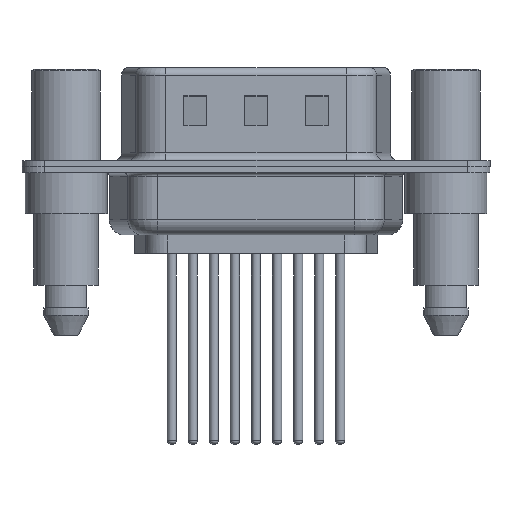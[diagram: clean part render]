
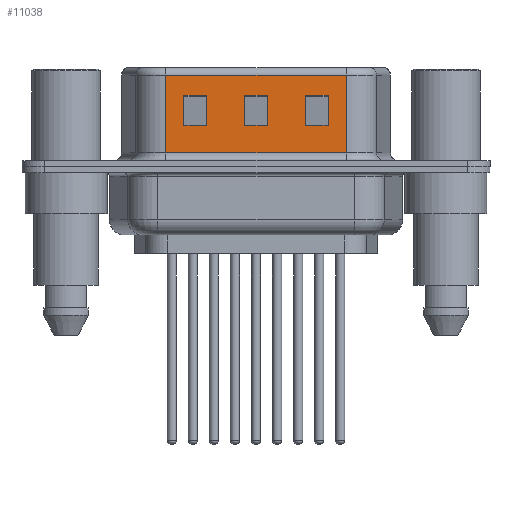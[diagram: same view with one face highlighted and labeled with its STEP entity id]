
A CAD part, front view. The second image highlights one B-rep face of the part: STEP entity #11038.
In plain terms, the highlighted planar face has unit normal (0, -1, 0).
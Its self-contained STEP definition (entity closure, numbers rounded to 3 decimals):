
#74 = CARTESIAN_POINT ( 'NONE',  ( 9.25, -4.55, 4.705 ) ) ;
#167 = CARTESIAN_POINT ( 'NONE',  ( 17.25, -4.55, 6.52 ) ) ;
#436 = LINE ( 'NONE', #4995, #13850 ) ;
#758 = VERTEX_POINT ( 'NONE', #74 ) ;
#816 = ORIENTED_EDGE ( 'NONE', *, *, #9312, .T. ) ;
#884 = VECTOR ( 'NONE', #4699, 1000. ) ;
#929 = VECTOR ( 'NONE', #10079, 1000. ) ;
#950 = DIRECTION ( 'NONE',  ( 0., 0., -1. ) ) ;
#968 = DIRECTION ( 'NONE',  ( -1., 0., 0. ) ) ;
#1068 = EDGE_CURVE ( 'NONE', #1913, #12412, #10161, .T. ) ;
#1203 = DIRECTION ( 'NONE',  ( 0., 0., -1. ) ) ;
#1407 = CARTESIAN_POINT ( 'NONE',  ( 18.451, -4.55, 0.9 ) ) ;
#1433 = VERTEX_POINT ( 'NONE', #2046 ) ;
#1436 = VECTOR ( 'NONE', #12580, 1000. ) ;
#1450 = VERTEX_POINT ( 'NONE', #7781 ) ;
#1588 = EDGE_LOOP ( 'NONE', ( #8142, #12219, #5133, #12017 ) ) ;
#1843 = EDGE_CURVE ( 'NONE', #12696, #6609, #7692, .T. ) ;
#1893 = ORIENTED_EDGE ( 'NONE', *, *, #9123, .T. ) ;
#1907 = EDGE_CURVE ( 'NONE', #1450, #7329, #2392, .T. ) ;
#1913 = VERTEX_POINT ( 'NONE', #11453 ) ;
#1971 = VECTOR ( 'NONE', #6741, 1000. ) ;
#2046 = CARTESIAN_POINT ( 'NONE',  ( 17.25, -4.55, 4.705 ) ) ;
#2392 = LINE ( 'NONE', #5786, #5528 ) ;
#2848 = VECTOR ( 'NONE', #13832, 1000. ) ;
#2907 = ORIENTED_EDGE ( 'NONE', *, *, #3967, .T. ) ;
#3003 = EDGE_CURVE ( 'NONE', #5905, #1450, #13193, .T. ) ;
#3876 = VECTOR ( 'NONE', #14158, 1000. ) ;
#3967 = EDGE_CURVE ( 'NONE', #9337, #12696, #13214, .T. ) ;
#4340 = CARTESIAN_POINT ( 'NONE',  ( 15.75, -4.55, 6.52 ) ) ;
#4435 = VERTEX_POINT ( 'NONE', #8905 ) ;
#4531 = AXIS2_PLACEMENT_3D ( 'NONE', #6543, #13302, #6613 ) ;
#4615 = EDGE_CURVE ( 'NONE', #1913, #10646, #9132, .T. ) ;
#4657 = VERTEX_POINT ( 'NONE', #8022 ) ;
#4660 = DIRECTION ( 'NONE',  ( 1., 0., 0. ) ) ;
#4699 = DIRECTION ( 'NONE',  ( -1., 0., 0. ) ) ;
#4855 = LINE ( 'NONE', #9362, #2848 ) ;
#4920 = DIRECTION ( 'NONE',  ( 1., 0., 0. ) ) ;
#4995 = CARTESIAN_POINT ( 'NONE',  ( 14.451, -4.55, 4.705 ) ) ;
#5128 = CARTESIAN_POINT ( 'NONE',  ( 7.75, -4.55, 4.705 ) ) ;
#5133 = ORIENTED_EDGE ( 'NONE', *, *, #3003, .T. ) ;
#5211 = CARTESIAN_POINT ( 'NONE',  ( 6.549, -4.55, 0.9 ) ) ;
#5231 = LINE ( 'NONE', #9727, #14067 ) ;
#5528 = VECTOR ( 'NONE', #6887, 1000. ) ;
#5719 = EDGE_CURVE ( 'NONE', #11653, #4657, #5231, .T. ) ;
#5736 = ORIENTED_EDGE ( 'NONE', *, *, #6155, .T. ) ;
#5747 = CARTESIAN_POINT ( 'NONE',  ( 18.451, -4.55, 6.02 ) ) ;
#5786 = CARTESIAN_POINT ( 'NONE',  ( 11.75, -4.55, 6.52 ) ) ;
#5815 = VECTOR ( 'NONE', #9989, 1000. ) ;
#5905 = VERTEX_POINT ( 'NONE', #6856 ) ;
#5963 = VECTOR ( 'NONE', #4660, 1000. ) ;
#6142 = VERTEX_POINT ( 'NONE', #9570 ) ;
#6155 = EDGE_CURVE ( 'NONE', #6609, #758, #436, .T. ) ;
#6403 = EDGE_CURVE ( 'NONE', #758, #9337, #13445, .T. ) ;
#6543 = CARTESIAN_POINT ( 'NONE',  ( 18.451, -4.55, 6.52 ) ) ;
#6609 = VERTEX_POINT ( 'NONE', #5128 ) ;
#6613 = DIRECTION ( 'NONE',  ( 0., 0., 1. ) ) ;
#6741 = DIRECTION ( 'NONE',  ( 0., 0., -1. ) ) ;
#6771 = ORIENTED_EDGE ( 'NONE', *, *, #4615, .T. ) ;
#6856 = CARTESIAN_POINT ( 'NONE',  ( 13.25, -4.55, 2.705 ) ) ;
#6887 = DIRECTION ( 'NONE',  ( 0., 0., 1. ) ) ;
#7236 = DIRECTION ( 'NONE',  ( -1., 0., 0. ) ) ;
#7329 = VERTEX_POINT ( 'NONE', #8925 ) ;
#7454 = EDGE_LOOP ( 'NONE', ( #8975, #2907, #9121, #5736 ) ) ;
#7455 = EDGE_CURVE ( 'NONE', #6142, #5905, #12531, .T. ) ;
#7569 = FACE_OUTER_BOUND ( 'NONE', #10349, .T. ) ;
#7645 = FACE_BOUND ( 'NONE', #8161, .T. ) ;
#7692 = LINE ( 'NONE', #9689, #3876 ) ;
#7725 = CARTESIAN_POINT ( 'NONE',  ( 6.549, -4.55, 6.02 ) ) ;
#7726 = LINE ( 'NONE', #4340, #11610 ) ;
#7781 = CARTESIAN_POINT ( 'NONE',  ( 11.75, -4.55, 2.705 ) ) ;
#8022 = CARTESIAN_POINT ( 'NONE',  ( 15.75, -4.55, 2.705 ) ) ;
#8142 = ORIENTED_EDGE ( 'NONE', *, *, #11652, .T. ) ;
#8161 = EDGE_LOOP ( 'NONE', ( #10404, #11479, #11809, #1893 ) ) ;
#8582 = VECTOR ( 'NONE', #950, 1000. ) ;
#8818 = PLANE ( 'NONE',  #4531 ) ;
#8836 = LINE ( 'NONE', #13319, #8582 ) ;
#8905 = CARTESIAN_POINT ( 'NONE',  ( 15.75, -4.55, 4.705 ) ) ;
#8925 = CARTESIAN_POINT ( 'NONE',  ( 11.75, -4.55, 4.705 ) ) ;
#8975 = ORIENTED_EDGE ( 'NONE', *, *, #6403, .T. ) ;
#9016 = CARTESIAN_POINT ( 'NONE',  ( 18.451, -4.55, 4.705 ) ) ;
#9059 = CARTESIAN_POINT ( 'NONE',  ( 18.451, -4.55, 0.9 ) ) ;
#9121 = ORIENTED_EDGE ( 'NONE', *, *, #1843, .T. ) ;
#9123 = EDGE_CURVE ( 'NONE', #4435, #1433, #4855, .T. ) ;
#9132 = LINE ( 'NONE', #5747, #884 ) ;
#9164 = CARTESIAN_POINT ( 'NONE',  ( 17.25, -4.55, 2.705 ) ) ;
#9312 = EDGE_CURVE ( 'NONE', #9717, #12412, #10302, .T. ) ;
#9337 = VERTEX_POINT ( 'NONE', #12365 ) ;
#9362 = CARTESIAN_POINT ( 'NONE',  ( 22.451, -4.55, 4.705 ) ) ;
#9376 = ORIENTED_EDGE ( 'NONE', *, *, #12620, .T. ) ;
#9570 = CARTESIAN_POINT ( 'NONE',  ( 13.25, -4.55, 4.705 ) ) ;
#9584 = VECTOR ( 'NONE', #10377, 1000. ) ;
#9689 = CARTESIAN_POINT ( 'NONE',  ( 7.75, -4.55, 6.52 ) ) ;
#9717 = VERTEX_POINT ( 'NONE', #5211 ) ;
#9727 = CARTESIAN_POINT ( 'NONE',  ( 22.451, -4.55, 2.705 ) ) ;
#9730 = VECTOR ( 'NONE', #968, 1000. ) ;
#9989 = DIRECTION ( 'NONE',  ( -1., 0., 0. ) ) ;
#10079 = DIRECTION ( 'NONE',  ( 0., 0., -1. ) ) ;
#10093 = CARTESIAN_POINT ( 'NONE',  ( 7.75, -4.55, 2.705 ) ) ;
#10126 = LINE ( 'NONE', #9016, #5963 ) ;
#10161 = LINE ( 'NONE', #11416, #9584 ) ;
#10302 = LINE ( 'NONE', #9059, #1436 ) ;
#10349 = EDGE_LOOP ( 'NONE', ( #14128, #6771, #9376, #816 ) ) ;
#10377 = DIRECTION ( 'NONE',  ( 0., 0., -1. ) ) ;
#10404 = ORIENTED_EDGE ( 'NONE', *, *, #11687, .T. ) ;
#10646 = VERTEX_POINT ( 'NONE', #7725 ) ;
#11038 = ADVANCED_FACE ( 'NONE', ( #13153, #7645, #14258, #7569 ), #8818, .F. ) ;
#11172 = CARTESIAN_POINT ( 'NONE',  ( 14.451, -4.55, 2.705 ) ) ;
#11416 = CARTESIAN_POINT ( 'NONE',  ( 18.451, -4.55, 6.52 ) ) ;
#11453 = CARTESIAN_POINT ( 'NONE',  ( 18.451, -4.55, 6.02 ) ) ;
#11479 = ORIENTED_EDGE ( 'NONE', *, *, #5719, .T. ) ;
#11610 = VECTOR ( 'NONE', #12225, 1000. ) ;
#11652 = EDGE_CURVE ( 'NONE', #7329, #6142, #10126, .T. ) ;
#11653 = VERTEX_POINT ( 'NONE', #9164 ) ;
#11687 = EDGE_CURVE ( 'NONE', #1433, #11653, #12331, .T. ) ;
#11809 = ORIENTED_EDGE ( 'NONE', *, *, #12707, .T. ) ;
#12017 = ORIENTED_EDGE ( 'NONE', *, *, #1907, .T. ) ;
#12219 = ORIENTED_EDGE ( 'NONE', *, *, #7455, .T. ) ;
#12225 = DIRECTION ( 'NONE',  ( 0., 0., 1. ) ) ;
#12331 = LINE ( 'NONE', #167, #1971 ) ;
#12365 = CARTESIAN_POINT ( 'NONE',  ( 9.25, -4.55, 2.705 ) ) ;
#12392 = CARTESIAN_POINT ( 'NONE',  ( 13.25, -4.55, 6.52 ) ) ;
#12412 = VERTEX_POINT ( 'NONE', #1407 ) ;
#12531 = LINE ( 'NONE', #12392, #13170 ) ;
#12580 = DIRECTION ( 'NONE',  ( 1., 0., 0. ) ) ;
#12620 = EDGE_CURVE ( 'NONE', #10646, #9717, #8836, .T. ) ;
#12696 = VERTEX_POINT ( 'NONE', #10093 ) ;
#12707 = EDGE_CURVE ( 'NONE', #4657, #4435, #7726, .T. ) ;
#13153 = FACE_BOUND ( 'NONE', #7454, .T. ) ;
#13170 = VECTOR ( 'NONE', #1203, 1000. ) ;
#13193 = LINE ( 'NONE', #13337, #9730 ) ;
#13214 = LINE ( 'NONE', #11172, #5815 ) ;
#13302 = DIRECTION ( 'NONE',  ( 0., 1., 0. ) ) ;
#13319 = CARTESIAN_POINT ( 'NONE',  ( 6.549, -4.55, 6.52 ) ) ;
#13337 = CARTESIAN_POINT ( 'NONE',  ( 18.451, -4.55, 2.705 ) ) ;
#13445 = LINE ( 'NONE', #13522, #929 ) ;
#13522 = CARTESIAN_POINT ( 'NONE',  ( 9.25, -4.55, 6.52 ) ) ;
#13832 = DIRECTION ( 'NONE',  ( 1., 0., 0. ) ) ;
#13850 = VECTOR ( 'NONE', #4920, 1000. ) ;
#14067 = VECTOR ( 'NONE', #7236, 1000. ) ;
#14128 = ORIENTED_EDGE ( 'NONE', *, *, #1068, .F. ) ;
#14158 = DIRECTION ( 'NONE',  ( 0., 0., 1. ) ) ;
#14258 = FACE_BOUND ( 'NONE', #1588, .T. ) ;
